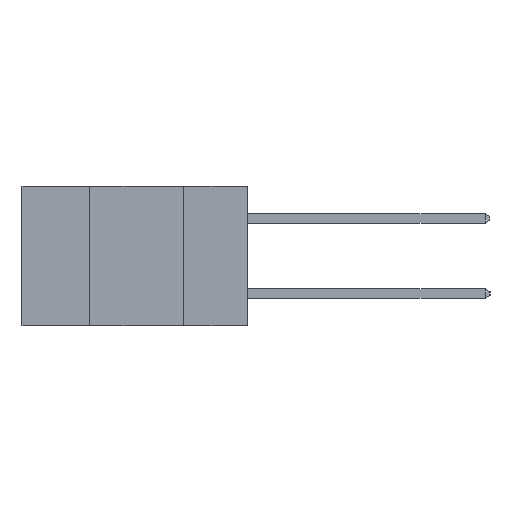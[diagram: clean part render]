
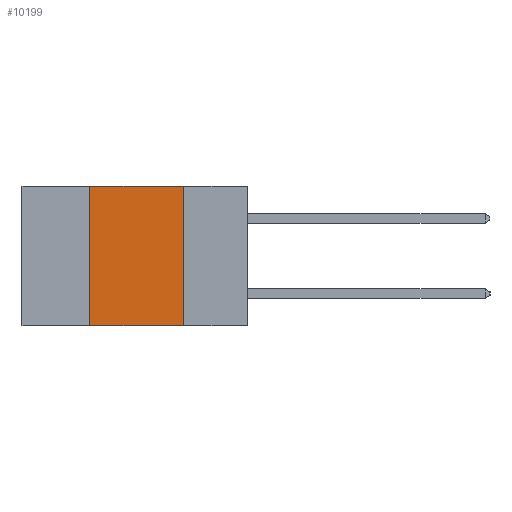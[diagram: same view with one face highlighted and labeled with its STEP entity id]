
A CAD part, left-side view. The second image highlights one B-rep face of the part: STEP entity #10199.
In plain terms, the highlighted planar face has unit normal (-1, 0, 0).
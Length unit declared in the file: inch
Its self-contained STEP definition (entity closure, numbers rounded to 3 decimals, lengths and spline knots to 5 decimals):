
#143 = CARTESIAN_POINT ( 'NONE',  ( 0., 0.17, -0.37 ) ) ;
#215 = CARTESIAN_POINT ( 'NONE',  ( 0., 0.42, 0. ) ) ;
#437 = CARTESIAN_POINT ( 'NONE',  ( 0., 0.6, 0. ) ) ;
#1791 = DIRECTION ( 'NONE',  ( 1., 0., 0. ) ) ;
#1819 = VERTEX_POINT ( 'NONE', #14127 ) ;
#2233 = ORIENTED_EDGE ( 'NONE', *, *, #3921, .F. ) ;
#2538 = LINE ( 'NONE', #5871, #12670 ) ;
#3694 = DIRECTION ( 'NONE',  ( 0., 0., 1. ) ) ;
#3921 = EDGE_CURVE ( 'NONE', #15274, #15913, #4652, .T. ) ;
#4245 = VECTOR ( 'NONE', #12666, 39.37008 ) ;
#4652 = LINE ( 'NONE', #143, #11244 ) ;
#4739 = FACE_OUTER_BOUND ( 'NONE', #10834, .T. ) ;
#4816 = EDGE_CURVE ( 'NONE', #10753, #15274, #2538, .T. ) ;
#5849 = DIRECTION ( 'NONE',  ( 0., -1., 0. ) ) ;
#5871 = CARTESIAN_POINT ( 'NONE',  ( 0., 0.6, 0. ) ) ;
#6150 = ORIENTED_EDGE ( 'NONE', *, *, #4816, .F. ) ;
#6280 = EDGE_CURVE ( 'NONE', #1819, #15913, #7750, .T. ) ;
#7016 = ORIENTED_EDGE ( 'NONE', *, *, #9189, .F. ) ;
#7750 = LINE ( 'NONE', #12721, #4245 ) ;
#7826 = ORIENTED_EDGE ( 'NONE', *, *, #6280, .T. ) ;
#8357 = PLANE ( 'NONE',  #11758 ) ;
#9189 = EDGE_CURVE ( 'NONE', #1819, #10753, #16126, .T. ) ;
#10199 = ADVANCED_FACE ( 'NONE', ( #4739 ), #8357, .F. ) ;
#10753 = VERTEX_POINT ( 'NONE', #215 ) ;
#10834 = EDGE_LOOP ( 'NONE', ( #2233, #6150, #7016, #7826 ) ) ;
#11006 = DIRECTION ( 'NONE',  ( 0., 0., -1. ) ) ;
#11244 = VECTOR ( 'NONE', #16674, 39.37008 ) ;
#11546 = CARTESIAN_POINT ( 'NONE',  ( 0., 0.17, -0.37 ) ) ;
#11597 = CARTESIAN_POINT ( 'NONE',  ( 0., 0.42, -0.37 ) ) ;
#11758 = AXIS2_PLACEMENT_3D ( 'NONE', #437, #1791, #11006 ) ;
#12666 = DIRECTION ( 'NONE',  ( 0., -1., 0. ) ) ;
#12670 = VECTOR ( 'NONE', #5849, 39.37008 ) ;
#12721 = CARTESIAN_POINT ( 'NONE',  ( 0., 0.6, -0.37 ) ) ;
#14127 = CARTESIAN_POINT ( 'NONE',  ( 0., 0.42, -0.37 ) ) ;
#15274 = VERTEX_POINT ( 'NONE', #16664 ) ;
#15742 = VECTOR ( 'NONE', #3694, 39.37008 ) ;
#15913 = VERTEX_POINT ( 'NONE', #11546 ) ;
#16126 = LINE ( 'NONE', #11597, #15742 ) ;
#16664 = CARTESIAN_POINT ( 'NONE',  ( 0., 0.17, 0. ) ) ;
#16674 = DIRECTION ( 'NONE',  ( 0., 0., -1. ) ) ;
